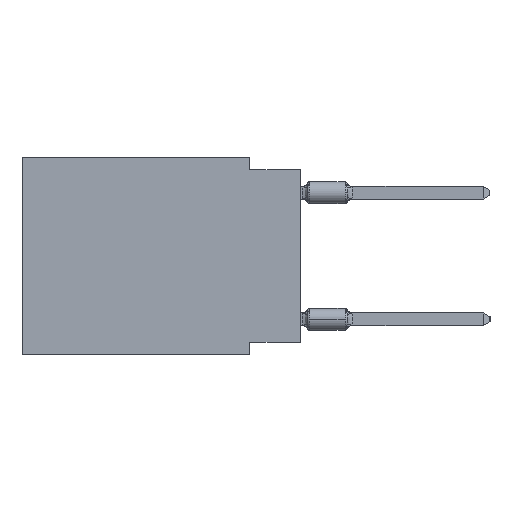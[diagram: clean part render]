
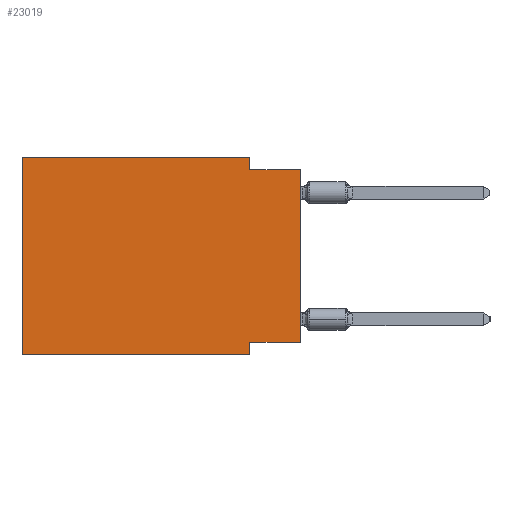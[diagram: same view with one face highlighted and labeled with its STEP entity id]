
A CAD part, left-side view. The second image highlights one B-rep face of the part: STEP entity #23019.
In plain terms, the highlighted planar face has unit normal (-1, 0, 0).
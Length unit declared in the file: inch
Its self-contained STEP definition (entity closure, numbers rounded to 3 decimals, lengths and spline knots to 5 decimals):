
#1921 = CARTESIAN_POINT ( 'NONE',  ( 0., 0.55, -0.39 ) ) ;
#2018 = ORIENTED_EDGE ( 'NONE', *, *, #14663, .F. ) ;
#2221 = ORIENTED_EDGE ( 'NONE', *, *, #5195, .F. ) ;
#2628 = LINE ( 'NONE', #16994, #44922 ) ;
#4697 = CARTESIAN_POINT ( 'NONE',  ( 0., 0.1, 0. ) ) ;
#5074 = DIRECTION ( 'NONE',  ( 1., 0., 0. ) ) ;
#5195 = EDGE_CURVE ( 'NONE', #27104, #22446, #28327, .T. ) ;
#5451 = LINE ( 'NONE', #1921, #14237 ) ;
#5737 = DIRECTION ( 'NONE',  ( 0., 0., -1. ) ) ;
#7482 = CARTESIAN_POINT ( 'NONE',  ( 0., 0., -0.365 ) ) ;
#8729 = EDGE_CURVE ( 'NONE', #38252, #18841, #14865, .T. ) ;
#9306 = FACE_OUTER_BOUND ( 'NONE', #22041, .T. ) ;
#9483 = ORIENTED_EDGE ( 'NONE', *, *, #8729, .F. ) ;
#10196 = CARTESIAN_POINT ( 'NONE',  ( 0., 0.1, -0.39 ) ) ;
#10267 = CARTESIAN_POINT ( 'NONE',  ( 0., 0.1, -0.39 ) ) ;
#11212 = CARTESIAN_POINT ( 'NONE',  ( 0., 0., 0. ) ) ;
#11316 = AXIS2_PLACEMENT_3D ( 'NONE', #30767, #5074, #30522 ) ;
#11552 = VECTOR ( 'NONE', #43179, 39.37008 ) ;
#12737 = EDGE_CURVE ( 'NONE', #18841, #39750, #17029, .T. ) ;
#13258 = VERTEX_POINT ( 'NONE', #24993 ) ;
#14237 = VECTOR ( 'NONE', #30909, 39.37008 ) ;
#14663 = EDGE_CURVE ( 'NONE', #13258, #27104, #33242, .T. ) ;
#14865 = LINE ( 'NONE', #37234, #37484 ) ;
#15062 = CARTESIAN_POINT ( 'NONE',  ( 0., 0.55, -0.39 ) ) ;
#15620 = EDGE_CURVE ( 'NONE', #36622, #26321, #33810, .T. ) ;
#16994 = CARTESIAN_POINT ( 'NONE',  ( 0., 0.55, 0. ) ) ;
#17029 = LINE ( 'NONE', #10196, #30345 ) ;
#18597 = EDGE_CURVE ( 'NONE', #26321, #13258, #2628, .T. ) ;
#18841 = VERTEX_POINT ( 'NONE', #30162 ) ;
#19009 = ORIENTED_EDGE ( 'NONE', *, *, #15620, .F. ) ;
#19345 = EDGE_CURVE ( 'NONE', #38252, #22446, #37751, .T. ) ;
#21108 = EDGE_CURVE ( 'NONE', #36622, #39750, #5451, .T. ) ;
#22041 = EDGE_LOOP ( 'NONE', ( #45605, #2221, #2018, #44191, #19009, #22585, #44793, #9483 ) ) ;
#22446 = VERTEX_POINT ( 'NONE', #37776 ) ;
#22585 = ORIENTED_EDGE ( 'NONE', *, *, #21108, .T. ) ;
#23019 = ADVANCED_FACE ( 'NONE', ( #9306 ), #37151, .F. ) ;
#23429 = CARTESIAN_POINT ( 'NONE',  ( 0., 0.55, 0. ) ) ;
#24644 = VECTOR ( 'NONE', #25588, 39.37008 ) ;
#24993 = CARTESIAN_POINT ( 'NONE',  ( 0., 0.1, 0. ) ) ;
#25588 = DIRECTION ( 'NONE',  ( 0., 0., 1. ) ) ;
#26321 = VERTEX_POINT ( 'NONE', #39744 ) ;
#27104 = VERTEX_POINT ( 'NONE', #39716 ) ;
#28327 = LINE ( 'NONE', #39180, #11552 ) ;
#29695 = DIRECTION ( 'NONE',  ( 0., 1., 0. ) ) ;
#30162 = CARTESIAN_POINT ( 'NONE',  ( 0., 0.1, -0.365 ) ) ;
#30251 = DIRECTION ( 'NONE',  ( 0., 0., 1. ) ) ;
#30345 = VECTOR ( 'NONE', #5737, 39.37008 ) ;
#30522 = DIRECTION ( 'NONE',  ( 0., 0., -1. ) ) ;
#30767 = CARTESIAN_POINT ( 'NONE',  ( 0., 0.55, 0. ) ) ;
#30909 = DIRECTION ( 'NONE',  ( 0., -1., 0. ) ) ;
#33242 = LINE ( 'NONE', #4697, #35757 ) ;
#33472 = DIRECTION ( 'NONE',  ( 0., 0., -1. ) ) ;
#33810 = LINE ( 'NONE', #23429, #46338 ) ;
#35757 = VECTOR ( 'NONE', #33472, 39.37008 ) ;
#36622 = VERTEX_POINT ( 'NONE', #15062 ) ;
#37151 = PLANE ( 'NONE',  #11316 ) ;
#37234 = CARTESIAN_POINT ( 'NONE',  ( 0., 0., -0.365 ) ) ;
#37484 = VECTOR ( 'NONE', #29695, 39.37008 ) ;
#37751 = LINE ( 'NONE', #11212, #24644 ) ;
#37776 = CARTESIAN_POINT ( 'NONE',  ( 0., 0., -0.025 ) ) ;
#38252 = VERTEX_POINT ( 'NONE', #7482 ) ;
#39180 = CARTESIAN_POINT ( 'NONE',  ( 0., 0., -0.025 ) ) ;
#39716 = CARTESIAN_POINT ( 'NONE',  ( 0., 0.1, -0.025 ) ) ;
#39744 = CARTESIAN_POINT ( 'NONE',  ( 0., 0.55, 0. ) ) ;
#39750 = VERTEX_POINT ( 'NONE', #10267 ) ;
#42239 = DIRECTION ( 'NONE',  ( 0., -1., 0. ) ) ;
#43179 = DIRECTION ( 'NONE',  ( 0., -1., 0. ) ) ;
#44191 = ORIENTED_EDGE ( 'NONE', *, *, #18597, .F. ) ;
#44793 = ORIENTED_EDGE ( 'NONE', *, *, #12737, .F. ) ;
#44922 = VECTOR ( 'NONE', #42239, 39.37008 ) ;
#45605 = ORIENTED_EDGE ( 'NONE', *, *, #19345, .T. ) ;
#46338 = VECTOR ( 'NONE', #30251, 39.37008 ) ;
